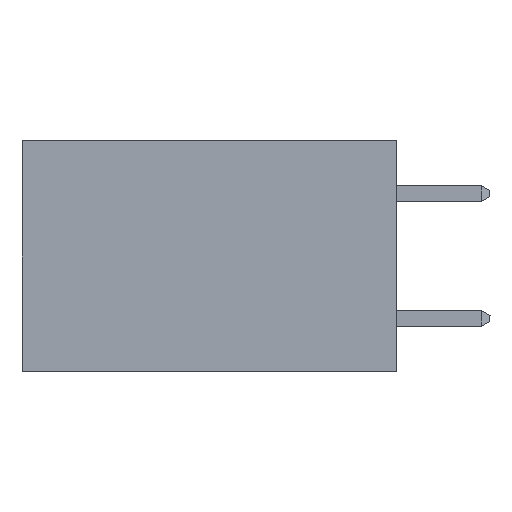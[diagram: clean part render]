
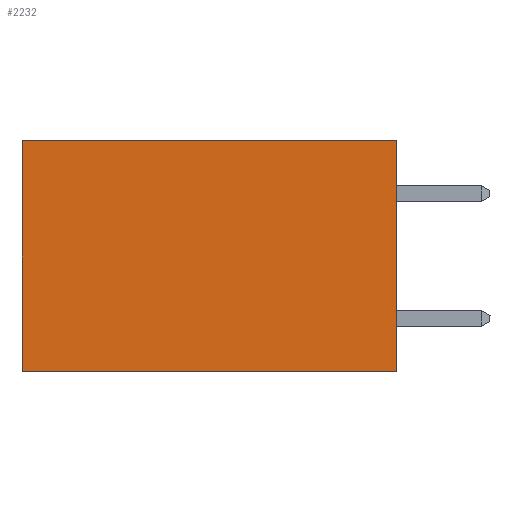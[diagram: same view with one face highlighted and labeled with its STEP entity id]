
A CAD part, left-side view. The second image highlights one B-rep face of the part: STEP entity #2232.
In plain terms, the highlighted planar face has unit normal (-1, 0, 0).
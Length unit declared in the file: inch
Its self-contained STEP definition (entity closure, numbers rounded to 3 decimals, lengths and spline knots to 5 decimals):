
#496 = AXIS2_PLACEMENT_3D ( 'NONE', #15379, #16935, #16692 ) ;
#596 = FACE_OUTER_BOUND ( 'NONE', #13608, .T. ) ;
#1406 = CARTESIAN_POINT ( 'NONE',  ( 0.2615, 0., -0.37 ) ) ;
#2195 = VERTEX_POINT ( 'NONE', #12900 ) ;
#2232 = ADVANCED_FACE ( 'NONE', ( #596 ), #7792, .F. ) ;
#3643 = CARTESIAN_POINT ( 'NONE',  ( 0.2615, 0., -0.37 ) ) ;
#4130 = ORIENTED_EDGE ( 'NONE', *, *, #20077, .T. ) ;
#4712 = VERTEX_POINT ( 'NONE', #16632 ) ;
#4830 = LINE ( 'NONE', #15980, #12031 ) ;
#5334 = EDGE_CURVE ( 'NONE', #4712, #11399, #5971, .T. ) ;
#5351 = DIRECTION ( 'NONE',  ( 0., 1., 0. ) ) ;
#5971 = LINE ( 'NONE', #6854, #14152 ) ;
#6798 = DIRECTION ( 'NONE',  ( 0., 0., -1. ) ) ;
#6854 = CARTESIAN_POINT ( 'NONE',  ( 0.2615, 0., -0.37 ) ) ;
#7190 = VECTOR ( 'NONE', #5351, 39.37008 ) ;
#7792 = PLANE ( 'NONE',  #496 ) ;
#11041 = DIRECTION ( 'NONE',  ( 0., 0., -1. ) ) ;
#11399 = VERTEX_POINT ( 'NONE', #1406 ) ;
#11503 = LINE ( 'NONE', #20555, #19604 ) ;
#12031 = VECTOR ( 'NONE', #12885, 39.37008 ) ;
#12543 = ORIENTED_EDGE ( 'NONE', *, *, #20560, .F. ) ;
#12664 = ORIENTED_EDGE ( 'NONE', *, *, #5334, .F. ) ;
#12885 = DIRECTION ( 'NONE',  ( 0., 1., 0. ) ) ;
#12900 = CARTESIAN_POINT ( 'NONE',  ( 0.2615, 0.6, 0. ) ) ;
#13608 = EDGE_LOOP ( 'NONE', ( #21058, #12543, #12664, #4130 ) ) ;
#14152 = VECTOR ( 'NONE', #6798, 39.37008 ) ;
#14532 = EDGE_CURVE ( 'NONE', #2195, #14631, #11503, .T. ) ;
#14631 = VERTEX_POINT ( 'NONE', #19389 ) ;
#15379 = CARTESIAN_POINT ( 'NONE',  ( 0.2615, 0., -0.37 ) ) ;
#15980 = CARTESIAN_POINT ( 'NONE',  ( 0.2615, 0., 0. ) ) ;
#16632 = CARTESIAN_POINT ( 'NONE',  ( 0.2615, 0., 0. ) ) ;
#16692 = DIRECTION ( 'NONE',  ( 0., 0., -1. ) ) ;
#16935 = DIRECTION ( 'NONE',  ( 1., 0., 0. ) ) ;
#19389 = CARTESIAN_POINT ( 'NONE',  ( 0.2615, 0.6, -0.37 ) ) ;
#19604 = VECTOR ( 'NONE', #11041, 39.37008 ) ;
#20077 = EDGE_CURVE ( 'NONE', #4712, #2195, #4830, .T. ) ;
#20084 = LINE ( 'NONE', #3643, #7190 ) ;
#20555 = CARTESIAN_POINT ( 'NONE',  ( 0.2615, 0.6, -0.37 ) ) ;
#20560 = EDGE_CURVE ( 'NONE', #11399, #14631, #20084, .T. ) ;
#21058 = ORIENTED_EDGE ( 'NONE', *, *, #14532, .T. ) ;
